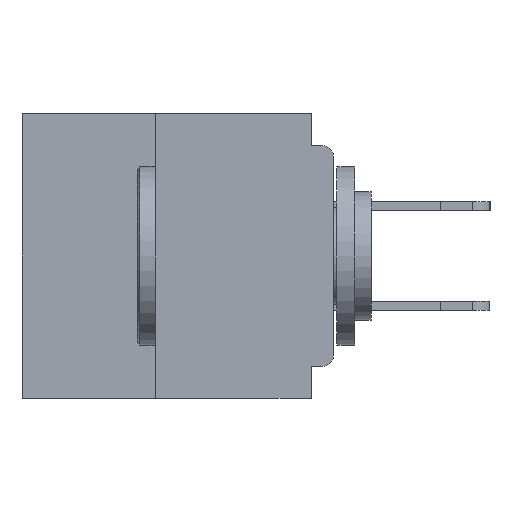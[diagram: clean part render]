
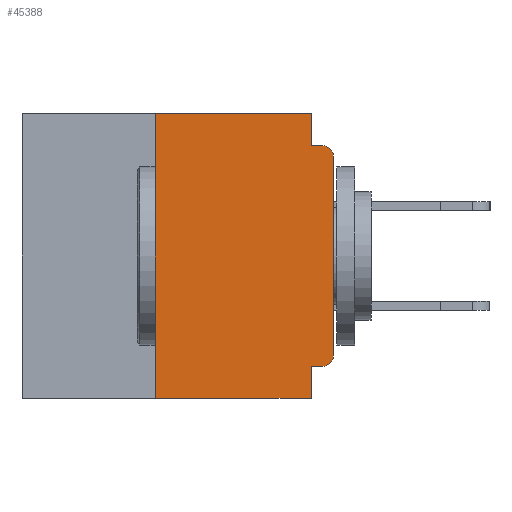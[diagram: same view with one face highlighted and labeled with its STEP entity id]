
A CAD part, left-side view. The second image highlights one B-rep face of the part: STEP entity #45388.
In plain terms, the highlighted planar face has unit normal (-1, 0, 0).
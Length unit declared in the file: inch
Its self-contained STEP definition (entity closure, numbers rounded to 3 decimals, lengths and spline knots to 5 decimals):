
#1043 = EDGE_LOOP ( 'NONE', ( #22561, #15461, #25851, #19829, #38464, #13821, #41729, #6690, #18238, #9994 ) ) ;
#3440 = LINE ( 'NONE', #22302, #12847 ) ;
#3872 = VECTOR ( 'NONE', #33319, 39.37008 ) ;
#4218 = DIRECTION ( 'NONE',  ( 0., -1., 0. ) ) ;
#4267 = CARTESIAN_POINT ( 'NONE',  ( 0., 0.25, 0. ) ) ;
#5246 = VERTEX_POINT ( 'NONE', #12149 ) ;
#5718 = VERTEX_POINT ( 'NONE', #19296 ) ;
#6690 = ORIENTED_EDGE ( 'NONE', *, *, #41300, .F. ) ;
#7516 = EDGE_CURVE ( 'NONE', #20394, #11642, #42565, .T. ) ;
#8196 = VERTEX_POINT ( 'NONE', #40211 ) ;
#9108 = CARTESIAN_POINT ( 'NONE',  ( 0., 0.031, 0. ) ) ;
#9936 = EDGE_CURVE ( 'NONE', #5246, #15136, #41598, .T. ) ;
#9994 = ORIENTED_EDGE ( 'NONE', *, *, #14103, .T. ) ;
#10969 = CARTESIAN_POINT ( 'NONE',  ( 0., 0.015, -0.06 ) ) ;
#10992 = PLANE ( 'NONE',  #23048 ) ;
#10995 = AXIS2_PLACEMENT_3D ( 'NONE', #10969, #35454, #14502 ) ;
#11642 = VERTEX_POINT ( 'NONE', #9108 ) ;
#12149 = CARTESIAN_POINT ( 'NONE',  ( 0., 0.25, -0.4 ) ) ;
#12292 = LINE ( 'NONE', #22266, #38045 ) ;
#12847 = VECTOR ( 'NONE', #43255, 39.37008 ) ;
#12879 = CARTESIAN_POINT ( 'NONE',  ( 0., 0.015, -0.34 ) ) ;
#13514 = CARTESIAN_POINT ( 'NONE',  ( 0., 0.015, -0.355 ) ) ;
#13588 = CARTESIAN_POINT ( 'NONE',  ( 0., 0.031, -0.4 ) ) ;
#13821 = ORIENTED_EDGE ( 'NONE', *, *, #19328, .F. ) ;
#14103 = EDGE_CURVE ( 'NONE', #26316, #8196, #43434, .T. ) ;
#14502 = DIRECTION ( 'NONE',  ( 0., 0., -1. ) ) ;
#15136 = VERTEX_POINT ( 'NONE', #13588 ) ;
#15318 = EDGE_CURVE ( 'NONE', #37714, #16962, #38009, .T. ) ;
#15461 = ORIENTED_EDGE ( 'NONE', *, *, #15318, .T. ) ;
#15653 = DIRECTION ( 'NONE',  ( 0., -1., 0. ) ) ;
#16421 = DIRECTION ( 'NONE',  ( 0., 0., -1. ) ) ;
#16732 = DIRECTION ( 'NONE',  ( 0., 0., -1. ) ) ;
#16962 = VERTEX_POINT ( 'NONE', #37789 ) ;
#18068 = DIRECTION ( 'NONE',  ( 1., 0., 0. ) ) ;
#18238 = ORIENTED_EDGE ( 'NONE', *, *, #35824, .F. ) ;
#19296 = CARTESIAN_POINT ( 'NONE',  ( 0., 0.031, -0.045 ) ) ;
#19328 = EDGE_CURVE ( 'NONE', #5246, #20394, #43124, .T. ) ;
#19560 = VERTEX_POINT ( 'NONE', #24419 ) ;
#19829 = ORIENTED_EDGE ( 'NONE', *, *, #21673, .F. ) ;
#20394 = VERTEX_POINT ( 'NONE', #4267 ) ;
#21129 = EDGE_CURVE ( 'NONE', #5718, #16962, #3440, .T. ) ;
#21380 = VECTOR ( 'NONE', #22678, 39.37008 ) ;
#21673 = EDGE_CURVE ( 'NONE', #11642, #5718, #12292, .T. ) ;
#22266 = CARTESIAN_POINT ( 'NONE',  ( 0., 0.031, 0. ) ) ;
#22302 = CARTESIAN_POINT ( 'NONE',  ( 0., 0., -0.045 ) ) ;
#22561 = ORIENTED_EDGE ( 'NONE', *, *, #28530, .T. ) ;
#22678 = DIRECTION ( 'NONE',  ( 0., 0., 1. ) ) ;
#22990 = VECTOR ( 'NONE', #4218, 39.37008 ) ;
#23048 = AXIS2_PLACEMENT_3D ( 'NONE', #39020, #18068, #42496 ) ;
#23136 = CARTESIAN_POINT ( 'NONE',  ( 0., 0., -0.06 ) ) ;
#24419 = CARTESIAN_POINT ( 'NONE',  ( 0., 0.031, -0.355 ) ) ;
#25252 = CARTESIAN_POINT ( 'NONE',  ( 0., 0.437, -0.4 ) ) ;
#25651 = LINE ( 'NONE', #37701, #33881 ) ;
#25851 = ORIENTED_EDGE ( 'NONE', *, *, #21129, .F. ) ;
#26316 = VERTEX_POINT ( 'NONE', #13514 ) ;
#26724 = VECTOR ( 'NONE', #33484, 39.37008 ) ;
#28530 = EDGE_CURVE ( 'NONE', #8196, #37714, #30685, .T. ) ;
#30685 = LINE ( 'NONE', #43448, #21380 ) ;
#33300 = VECTOR ( 'NONE', #15653, 39.37008 ) ;
#33319 = DIRECTION ( 'NONE',  ( 0., 1., 0. ) ) ;
#33484 = DIRECTION ( 'NONE',  ( 0., 0., 1. ) ) ;
#33881 = VECTOR ( 'NONE', #16732, 39.37008 ) ;
#34142 = AXIS2_PLACEMENT_3D ( 'NONE', #12879, #37380, #16421 ) ;
#35454 = DIRECTION ( 'NONE',  ( -1., 0., 0. ) ) ;
#35824 = EDGE_CURVE ( 'NONE', #26316, #19560, #40082, .T. ) ;
#36599 = CARTESIAN_POINT ( 'NONE',  ( 0., 0.437, 0. ) ) ;
#36663 = CARTESIAN_POINT ( 'NONE',  ( 0., 0., -0.355 ) ) ;
#36992 = CARTESIAN_POINT ( 'NONE',  ( 0., 0.25, -0.4 ) ) ;
#37380 = DIRECTION ( 'NONE',  ( -1., 0., 0. ) ) ;
#37701 = CARTESIAN_POINT ( 'NONE',  ( 0., 0.031, -0.4 ) ) ;
#37714 = VERTEX_POINT ( 'NONE', #23136 ) ;
#37789 = CARTESIAN_POINT ( 'NONE',  ( 0., 0.015, -0.045 ) ) ;
#38009 = CIRCLE ( 'NONE', #10995, 0.015 ) ;
#38045 = VECTOR ( 'NONE', #39716, 39.37008 ) ;
#38396 = FACE_OUTER_BOUND ( 'NONE', #1043, .T. ) ;
#38464 = ORIENTED_EDGE ( 'NONE', *, *, #7516, .F. ) ;
#39020 = CARTESIAN_POINT ( 'NONE',  ( 0., 0.437, 0. ) ) ;
#39716 = DIRECTION ( 'NONE',  ( 0., 0., -1. ) ) ;
#40082 = LINE ( 'NONE', #36663, #3872 ) ;
#40211 = CARTESIAN_POINT ( 'NONE',  ( 0., 0., -0.34 ) ) ;
#41300 = EDGE_CURVE ( 'NONE', #19560, #15136, #25651, .T. ) ;
#41598 = LINE ( 'NONE', #25252, #22990 ) ;
#41729 = ORIENTED_EDGE ( 'NONE', *, *, #9936, .T. ) ;
#42496 = DIRECTION ( 'NONE',  ( 0., 0., -1. ) ) ;
#42565 = LINE ( 'NONE', #36599, #33300 ) ;
#43124 = LINE ( 'NONE', #36992, #26724 ) ;
#43255 = DIRECTION ( 'NONE',  ( 0., -1., 0. ) ) ;
#43434 = CIRCLE ( 'NONE', #34142, 0.015 ) ;
#43448 = CARTESIAN_POINT ( 'NONE',  ( 0., 0., 0. ) ) ;
#45388 = ADVANCED_FACE ( 'NONE', ( #38396 ), #10992, .F. ) ;
